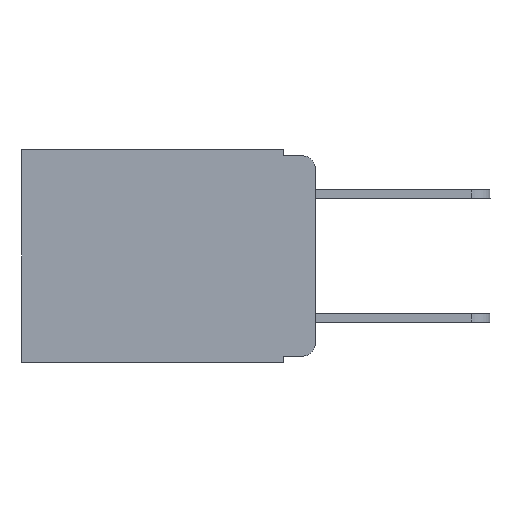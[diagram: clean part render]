
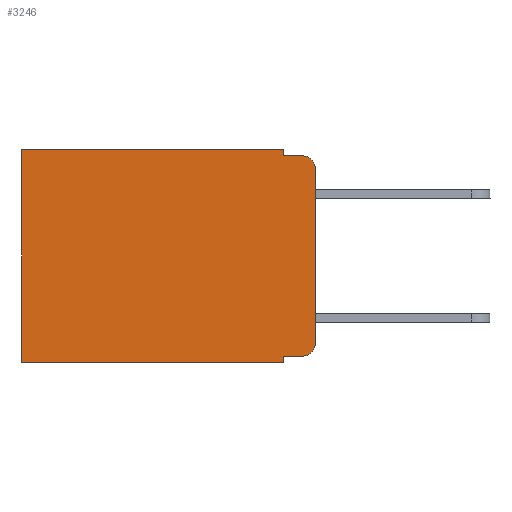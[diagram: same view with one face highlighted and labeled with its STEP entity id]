
A CAD part, left-side view. The second image highlights one B-rep face of the part: STEP entity #3246.
In plain terms, the highlighted planar face has unit normal (-1, 0, 0).
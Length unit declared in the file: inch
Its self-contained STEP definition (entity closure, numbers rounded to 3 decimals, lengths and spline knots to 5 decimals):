
#86 = EDGE_CURVE ( 'NONE', #8862, #2874, #4779, .T. ) ;
#156 = FACE_OUTER_BOUND ( 'NONE', #3366, .T. ) ;
#209 = CARTESIAN_POINT ( 'NONE',  ( 0.298, 0., 0. ) ) ;
#224 = VERTEX_POINT ( 'NONE', #9040 ) ;
#355 = ORIENTED_EDGE ( 'NONE', *, *, #6748, .T. ) ;
#579 = VERTEX_POINT ( 'NONE', #1389 ) ;
#746 = AXIS2_PLACEMENT_3D ( 'NONE', #7119, #2716, #3434 ) ;
#827 = CARTESIAN_POINT ( 'NONE',  ( 0.298, 0.051, 0. ) ) ;
#1010 = CARTESIAN_POINT ( 'NONE',  ( 0.298, 0., 0. ) ) ;
#1039 = DIRECTION ( 'NONE',  ( 1., 0., 0. ) ) ;
#1259 = ORIENTED_EDGE ( 'NONE', *, *, #2944, .T. ) ;
#1289 = DIRECTION ( 'NONE',  ( -1., 0., 0. ) ) ;
#1389 = CARTESIAN_POINT ( 'NONE',  ( 0.298, 0., -0.313 ) ) ;
#1737 = ORIENTED_EDGE ( 'NONE', *, *, #2635, .F. ) ;
#1819 = LINE ( 'NONE', #7245, #2040 ) ;
#1876 = DIRECTION ( 'NONE',  ( 0., 1., 0. ) ) ;
#1892 = EDGE_CURVE ( 'NONE', #7669, #8862, #2216, .T. ) ;
#2040 = VECTOR ( 'NONE', #2163, 39.37008 ) ;
#2163 = DIRECTION ( 'NONE',  ( 0., 1., 0. ) ) ;
#2216 = LINE ( 'NONE', #827, #5301 ) ;
#2635 = EDGE_CURVE ( 'NONE', #7241, #579, #5876, .T. ) ;
#2716 = DIRECTION ( 'NONE',  ( -1., 0., 0. ) ) ;
#2825 = VECTOR ( 'NONE', #9418, 39.37008 ) ;
#2874 = VERTEX_POINT ( 'NONE', #5659 ) ;
#2944 = EDGE_CURVE ( 'NONE', #224, #579, #7839, .T. ) ;
#3151 = DIRECTION ( 'NONE',  ( 0., 0., -1. ) ) ;
#3210 = PLANE ( 'NONE',  #8974 ) ;
#3246 = ADVANCED_FACE ( 'NONE', ( #156 ), #3210, .F. ) ;
#3260 = LINE ( 'NONE', #8178, #7423 ) ;
#3285 = CARTESIAN_POINT ( 'NONE',  ( 0.298, 0.051, 0. ) ) ;
#3366 = EDGE_LOOP ( 'NONE', ( #1737, #8083, #8875, #5635, #9353, #7876, #6211, #8205, #355, #1259 ) ) ;
#3425 = CARTESIAN_POINT ( 'NONE',  ( 0.298, 0., -0.343 ) ) ;
#3434 = DIRECTION ( 'NONE',  ( 0., 0., -1. ) ) ;
#3500 = EDGE_CURVE ( 'NONE', #7241, #8211, #5284, .T. ) ;
#3571 = CARTESIAN_POINT ( 'NONE',  ( 0.298, 0.051, -0.343 ) ) ;
#3802 = VECTOR ( 'NONE', #3999, 39.37008 ) ;
#3858 = CARTESIAN_POINT ( 'NONE',  ( 0.298, 0.051, -0.333 ) ) ;
#3923 = CARTESIAN_POINT ( 'NONE',  ( 0.298, 0.051, 0. ) ) ;
#3965 = CARTESIAN_POINT ( 'NONE',  ( 0.298, 0.473, 0. ) ) ;
#3990 = DIRECTION ( 'NONE',  ( 0., 0., -1. ) ) ;
#3999 = DIRECTION ( 'NONE',  ( 0., 0., -1. ) ) ;
#4550 = VECTOR ( 'NONE', #1876, 39.37008 ) ;
#4707 = VERTEX_POINT ( 'NONE', #3285 ) ;
#4779 = LINE ( 'NONE', #3425, #4550 ) ;
#4877 = CARTESIAN_POINT ( 'NONE',  ( 0.298, 0.051, -0.01 ) ) ;
#5195 = VERTEX_POINT ( 'NONE', #3965 ) ;
#5284 = CIRCLE ( 'NONE', #6109, 0.02 ) ;
#5301 = VECTOR ( 'NONE', #5965, 39.37008 ) ;
#5635 = ORIENTED_EDGE ( 'NONE', *, *, #5824, .F. ) ;
#5659 = CARTESIAN_POINT ( 'NONE',  ( 0.298, 0.473, -0.343 ) ) ;
#5742 = DIRECTION ( 'NONE',  ( 0., 0., -1. ) ) ;
#5824 = EDGE_CURVE ( 'NONE', #4707, #7399, #8916, .T. ) ;
#5827 = CARTESIAN_POINT ( 'NONE',  ( 0.298, 0.051, -0.333 ) ) ;
#5876 = LINE ( 'NONE', #209, #3802 ) ;
#5965 = DIRECTION ( 'NONE',  ( 0., 0., -1. ) ) ;
#6036 = LINE ( 'NONE', #4877, #8450 ) ;
#6109 = AXIS2_PLACEMENT_3D ( 'NONE', #7923, #1289, #5742 ) ;
#6211 = ORIENTED_EDGE ( 'NONE', *, *, #86, .F. ) ;
#6690 = EDGE_CURVE ( 'NONE', #7399, #8211, #6036, .T. ) ;
#6748 = EDGE_CURVE ( 'NONE', #7669, #224, #8671, .T. ) ;
#6945 = EDGE_CURVE ( 'NONE', #5195, #2874, #3260, .T. ) ;
#7119 = CARTESIAN_POINT ( 'NONE',  ( 0.298, 0.02, -0.313 ) ) ;
#7241 = VERTEX_POINT ( 'NONE', #7768 ) ;
#7245 = CARTESIAN_POINT ( 'NONE',  ( 0.298, 0., 0. ) ) ;
#7310 = CARTESIAN_POINT ( 'NONE',  ( 0.298, 0.051, -0.01 ) ) ;
#7395 = EDGE_CURVE ( 'NONE', #4707, #5195, #1819, .T. ) ;
#7399 = VERTEX_POINT ( 'NONE', #7310 ) ;
#7423 = VECTOR ( 'NONE', #8148, 39.37008 ) ;
#7669 = VERTEX_POINT ( 'NONE', #3858 ) ;
#7768 = CARTESIAN_POINT ( 'NONE',  ( 0.298, 0., -0.03 ) ) ;
#7839 = CIRCLE ( 'NONE', #746, 0.02 ) ;
#7873 = DIRECTION ( 'NONE',  ( 0., -1., 0. ) ) ;
#7876 = ORIENTED_EDGE ( 'NONE', *, *, #6945, .T. ) ;
#7923 = CARTESIAN_POINT ( 'NONE',  ( 0.298, 0.02, -0.03 ) ) ;
#8083 = ORIENTED_EDGE ( 'NONE', *, *, #3500, .T. ) ;
#8148 = DIRECTION ( 'NONE',  ( 0., 0., -1. ) ) ;
#8178 = CARTESIAN_POINT ( 'NONE',  ( 0.298, 0.473, 0. ) ) ;
#8205 = ORIENTED_EDGE ( 'NONE', *, *, #1892, .F. ) ;
#8211 = VERTEX_POINT ( 'NONE', #8258 ) ;
#8258 = CARTESIAN_POINT ( 'NONE',  ( 0.298, 0.02, -0.01 ) ) ;
#8450 = VECTOR ( 'NONE', #7873, 39.37008 ) ;
#8671 = LINE ( 'NONE', #5827, #2825 ) ;
#8688 = VECTOR ( 'NONE', #3151, 39.37008 ) ;
#8862 = VERTEX_POINT ( 'NONE', #3571 ) ;
#8875 = ORIENTED_EDGE ( 'NONE', *, *, #6690, .F. ) ;
#8916 = LINE ( 'NONE', #3923, #8688 ) ;
#8974 = AXIS2_PLACEMENT_3D ( 'NONE', #1010, #1039, #3990 ) ;
#9040 = CARTESIAN_POINT ( 'NONE',  ( 0.298, 0.02, -0.333 ) ) ;
#9353 = ORIENTED_EDGE ( 'NONE', *, *, #7395, .T. ) ;
#9418 = DIRECTION ( 'NONE',  ( 0., -1., 0. ) ) ;
